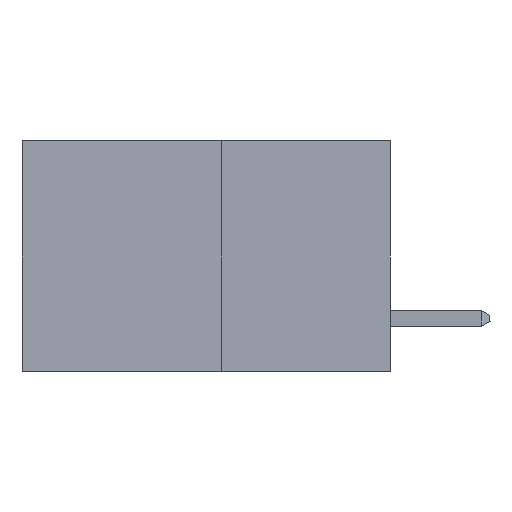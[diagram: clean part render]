
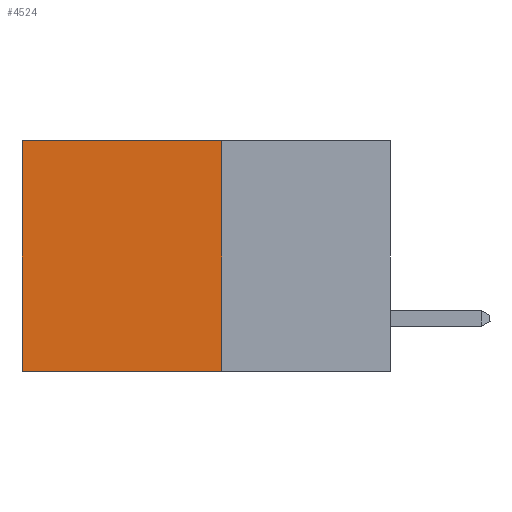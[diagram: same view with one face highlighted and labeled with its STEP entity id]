
A CAD part, left-side view. The second image highlights one B-rep face of the part: STEP entity #4524.
In plain terms, the highlighted planar face has unit normal (-1, 0, 0).
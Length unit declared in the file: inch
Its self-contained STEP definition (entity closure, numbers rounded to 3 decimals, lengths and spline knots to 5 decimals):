
#703 = VECTOR ( 'NONE', #10991, 39.37008 ) ;
#1864 = VECTOR ( 'NONE', #12879, 39.37008 ) ;
#3561 = CARTESIAN_POINT ( 'NONE',  ( 0.277, 0.27, -0.37 ) ) ;
#3974 = ORIENTED_EDGE ( 'NONE', *, *, #22901, .F. ) ;
#4524 = ADVANCED_FACE ( 'NONE', ( #16171 ), #21133, .F. ) ;
#5612 = LINE ( 'NONE', #3561, #703 ) ;
#7172 = VERTEX_POINT ( 'NONE', #16911 ) ;
#7321 = EDGE_CURVE ( 'NONE', #21791, #8121, #22256, .T. ) ;
#7460 = CARTESIAN_POINT ( 'NONE',  ( 0.277, 0.27, 0. ) ) ;
#8025 = ORIENTED_EDGE ( 'NONE', *, *, #10317, .T. ) ;
#8082 = VECTOR ( 'NONE', #8120, 39.37008 ) ;
#8120 = DIRECTION ( 'NONE',  ( 0., 0., -1. ) ) ;
#8121 = VERTEX_POINT ( 'NONE', #14071 ) ;
#8306 = ORIENTED_EDGE ( 'NONE', *, *, #7321, .T. ) ;
#8337 = CARTESIAN_POINT ( 'NONE',  ( 0.277, 0.59, -0.37 ) ) ;
#8339 = LINE ( 'NONE', #18206, #12648 ) ;
#10050 = ORIENTED_EDGE ( 'NONE', *, *, #19779, .F. ) ;
#10317 = EDGE_CURVE ( 'NONE', #21105, #21791, #10577, .T. ) ;
#10404 = EDGE_LOOP ( 'NONE', ( #8306, #3974, #10050, #8025 ) ) ;
#10577 = LINE ( 'NONE', #12930, #1864 ) ;
#10991 = DIRECTION ( 'NONE',  ( 0., 0., -1. ) ) ;
#11088 = DIRECTION ( 'NONE',  ( 0., 1., 0. ) ) ;
#12648 = VECTOR ( 'NONE', #11088, 39.37008 ) ;
#12879 = DIRECTION ( 'NONE',  ( 0., 1., 0. ) ) ;
#12930 = CARTESIAN_POINT ( 'NONE',  ( 0.277, 0.27, 0. ) ) ;
#14071 = CARTESIAN_POINT ( 'NONE',  ( 0.277, 0.59, -0.37 ) ) ;
#16171 = FACE_OUTER_BOUND ( 'NONE', #10404, .T. ) ;
#16183 = DIRECTION ( 'NONE',  ( 0., 0., -1. ) ) ;
#16347 = DIRECTION ( 'NONE',  ( 1., 0., 0. ) ) ;
#16911 = CARTESIAN_POINT ( 'NONE',  ( 0.277, 0.27, -0.37 ) ) ;
#18206 = CARTESIAN_POINT ( 'NONE',  ( 0.277, 0.27, -0.37 ) ) ;
#18743 = AXIS2_PLACEMENT_3D ( 'NONE', #21155, #16347, #16183 ) ;
#19779 = EDGE_CURVE ( 'NONE', #21105, #7172, #5612, .T. ) ;
#21105 = VERTEX_POINT ( 'NONE', #7460 ) ;
#21133 = PLANE ( 'NONE',  #18743 ) ;
#21155 = CARTESIAN_POINT ( 'NONE',  ( 0.277, 0.27, -0.37 ) ) ;
#21791 = VERTEX_POINT ( 'NONE', #21849 ) ;
#21849 = CARTESIAN_POINT ( 'NONE',  ( 0.277, 0.59, 0. ) ) ;
#22256 = LINE ( 'NONE', #8337, #8082 ) ;
#22901 = EDGE_CURVE ( 'NONE', #7172, #8121, #8339, .T. ) ;
